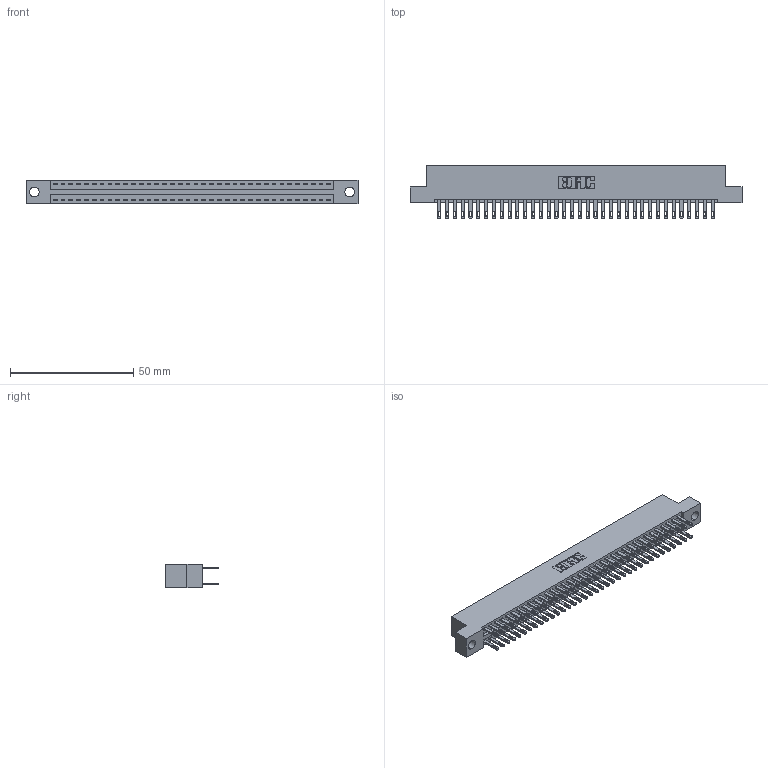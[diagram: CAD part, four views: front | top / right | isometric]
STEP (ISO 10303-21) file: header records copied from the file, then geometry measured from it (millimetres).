
FILE_DESCRIPTION (( 'STEP AP203' ), '1' );
FILE_NAME ('346-072-500-204.STEP', '2022-05-24T22:53:12', ( '' ), ( '' ), 'SwSTEP 2.0', 'SolidWorks 2020', '' );
FILE_SCHEMA (( 'CONFIG_CONTROL_DESIGN' ));
Length unit declared in the file: inch
Products named in the file (3): 346-072-500-204; 346 Part_Flush Mounting Lugs - 0.156 Dia-TH; 345-292-001_345-293-100
Assembly tree (73 placements, depth 2):
  346-072-500-204
    346 Part_Flush Mounting Lugs - 0.156 Dia-TH
    345-292-001_345-293-100  x72
Bounding box: 134.87 x 21.84 x 9.4 mm (x, y, z)
Volume: 13219.4 mm3; surface area: 18678.1 mm2
Topology: 73 solids, 73 shells, 3592 faces, 10949 edges, 7298 vertices
Faces by surface type: plane 2178, cylinder 1414
Entity records: 24651 total; most frequent: CARTESIAN_POINT 4074, ORIENTED_EDGE 4006, DIRECTION 3643, EDGE_CURVE 2003, LINE 1723, VECTOR 1723, VERTEX_POINT 1334, AXIS2_PLACEMENT_3D 960
